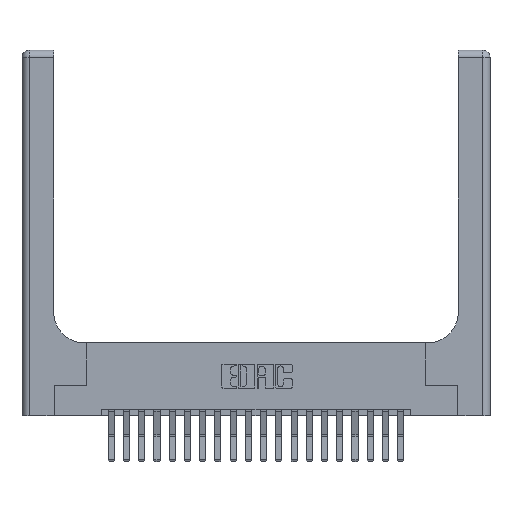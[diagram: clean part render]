
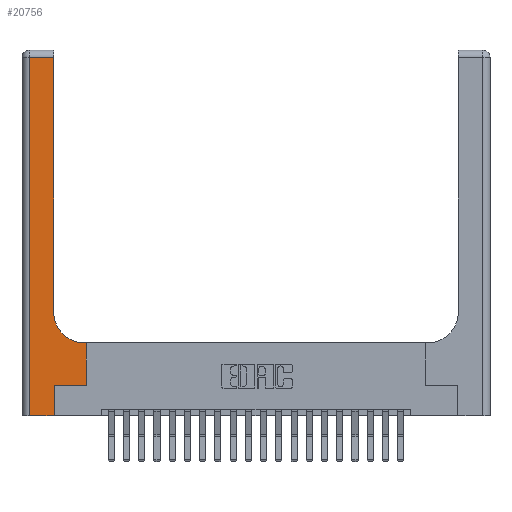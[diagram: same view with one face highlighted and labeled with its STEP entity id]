
A CAD part, top view. The second image highlights one B-rep face of the part: STEP entity #20756.
In plain terms, the highlighted planar face has unit normal (0, 0, 1).
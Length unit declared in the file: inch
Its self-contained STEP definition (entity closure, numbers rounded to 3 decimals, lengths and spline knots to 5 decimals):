
#89 = LINE ( 'NONE', #15101, #6809 ) ;
#337 = VECTOR ( 'NONE', #10274, 39.37008 ) ;
#774 = CARTESIAN_POINT ( 'NONE',  ( 0., 3., 0.37 ) ) ;
#1192 = EDGE_CURVE ( 'NONE', #19767, #1835, #10230, .T. ) ;
#1304 = VERTEX_POINT ( 'NONE', #4001 ) ;
#1382 = LINE ( 'NONE', #2144, #337 ) ;
#1524 = VERTEX_POINT ( 'NONE', #2040 ) ;
#1663 = VECTOR ( 'NONE', #15483, 39.37008 ) ;
#1835 = VERTEX_POINT ( 'NONE', #1923 ) ;
#1923 = CARTESIAN_POINT ( 'NONE',  ( 0.26, 0.85, 0.37 ) ) ;
#1961 = VECTOR ( 'NONE', #5392, 39.37008 ) ;
#2040 = CARTESIAN_POINT ( 'NONE',  ( 0.265, 0.25, 0.37 ) ) ;
#2084 = CARTESIAN_POINT ( 'NONE',  ( 0.265, 0., 0.37 ) ) ;
#2144 = CARTESIAN_POINT ( 'NONE',  ( 0., 0., 0.37 ) ) ;
#2389 = LINE ( 'NONE', #8883, #14966 ) ;
#3024 = ORIENTED_EDGE ( 'NONE', *, *, #19843, .T. ) ;
#3281 = EDGE_CURVE ( 'NONE', #1304, #16478, #4463, .T. ) ;
#3885 = ORIENTED_EDGE ( 'NONE', *, *, #8277, .T. ) ;
#4001 = CARTESIAN_POINT ( 'NONE',  ( 0.528, 0.25, 0.37 ) ) ;
#4047 = VECTOR ( 'NONE', #20188, 39.37008 ) ;
#4308 = EDGE_CURVE ( 'NONE', #13788, #12608, #2389, .T. ) ;
#4463 = LINE ( 'NONE', #16210, #19872 ) ;
#4501 = DIRECTION ( 'NONE',  ( 0., 1., 0. ) ) ;
#4838 = ORIENTED_EDGE ( 'NONE', *, *, #19431, .T. ) ;
#4858 = CARTESIAN_POINT ( 'NONE',  ( 0.51, 0.6, 0.37 ) ) ;
#5392 = DIRECTION ( 'NONE',  ( 0., 1., 0. ) ) ;
#6809 = VECTOR ( 'NONE', #13540, 39.37008 ) ;
#6857 = LINE ( 'NONE', #2084, #1961 ) ;
#6874 = LINE ( 'NONE', #20128, #4047 ) ;
#7096 = DIRECTION ( 'NONE',  ( 0., -1., 0. ) ) ;
#7355 = CARTESIAN_POINT ( 'NONE',  ( 0.26, 0.6, 0.37 ) ) ;
#8277 = EDGE_CURVE ( 'NONE', #1524, #1304, #6874, .T. ) ;
#8837 = EDGE_CURVE ( 'NONE', #13889, #1524, #6857, .T. ) ;
#8883 = CARTESIAN_POINT ( 'NONE',  ( 0.06, 3., 0.37 ) ) ;
#9096 = ORIENTED_EDGE ( 'NONE', *, *, #1192, .T. ) ;
#9409 = DIRECTION ( 'NONE',  ( 0., 0., -1. ) ) ;
#10230 = CIRCLE ( 'NONE', #12477, 0.25 ) ;
#10274 = DIRECTION ( 'NONE',  ( 1., 0., 0. ) ) ;
#10662 = DIRECTION ( 'NONE',  ( -1., 0., 0. ) ) ;
#10833 = DIRECTION ( 'NONE',  ( 1., 0., 0. ) ) ;
#10998 = CARTESIAN_POINT ( 'NONE',  ( 0.265, 0., 0.37 ) ) ;
#11542 = ORIENTED_EDGE ( 'NONE', *, *, #3281, .T. ) ;
#11955 = CARTESIAN_POINT ( 'NONE',  ( 0.26, 2.94, 0.37 ) ) ;
#12282 = DIRECTION ( 'NONE',  ( -1., 0., 0. ) ) ;
#12438 = CARTESIAN_POINT ( 'NONE',  ( 0.06, 0., 0.37 ) ) ;
#12477 = AXIS2_PLACEMENT_3D ( 'NONE', #15997, #9409, #10833 ) ;
#12608 = VERTEX_POINT ( 'NONE', #12438 ) ;
#12670 = VECTOR ( 'NONE', #10662, 39.37008 ) ;
#13058 = CARTESIAN_POINT ( 'NONE',  ( 0.528, 0.6, 0.37 ) ) ;
#13449 = LINE ( 'NONE', #7355, #12670 ) ;
#13540 = DIRECTION ( 'NONE',  ( -1., 0., 0. ) ) ;
#13788 = VERTEX_POINT ( 'NONE', #20417 ) ;
#13889 = VERTEX_POINT ( 'NONE', #10998 ) ;
#14966 = VECTOR ( 'NONE', #7096, 39.37008 ) ;
#15077 = ORIENTED_EDGE ( 'NONE', *, *, #17328, .T. ) ;
#15101 = CARTESIAN_POINT ( 'NONE',  ( 0., 2.94, 0.37 ) ) ;
#15345 = CARTESIAN_POINT ( 'NONE',  ( 0.26, 3., 0.37 ) ) ;
#15483 = DIRECTION ( 'NONE',  ( 0., 1., 0. ) ) ;
#15508 = PLANE ( 'NONE',  #19569 ) ;
#15997 = CARTESIAN_POINT ( 'NONE',  ( 0.51, 0.85, 0.37 ) ) ;
#16210 = CARTESIAN_POINT ( 'NONE',  ( 0.528, 0.25, 0.37 ) ) ;
#16283 = FACE_OUTER_BOUND ( 'NONE', #16352, .T. ) ;
#16352 = EDGE_LOOP ( 'NONE', ( #4838, #3024, #18745, #17567, #18770, #3885, #11542, #15077, #9096 ) ) ;
#16478 = VERTEX_POINT ( 'NONE', #13058 ) ;
#16623 = EDGE_CURVE ( 'NONE', #12608, #13889, #1382, .T. ) ;
#17117 = VERTEX_POINT ( 'NONE', #11955 ) ;
#17149 = DIRECTION ( 'NONE',  ( 0., 0., -1. ) ) ;
#17328 = EDGE_CURVE ( 'NONE', #16478, #19767, #13449, .T. ) ;
#17567 = ORIENTED_EDGE ( 'NONE', *, *, #16623, .T. ) ;
#18745 = ORIENTED_EDGE ( 'NONE', *, *, #4308, .T. ) ;
#18770 = ORIENTED_EDGE ( 'NONE', *, *, #8837, .T. ) ;
#19116 = LINE ( 'NONE', #15345, #1663 ) ;
#19431 = EDGE_CURVE ( 'NONE', #1835, #17117, #19116, .T. ) ;
#19569 = AXIS2_PLACEMENT_3D ( 'NONE', #774, #17149, #12282 ) ;
#19767 = VERTEX_POINT ( 'NONE', #4858 ) ;
#19843 = EDGE_CURVE ( 'NONE', #17117, #13788, #89, .T. ) ;
#19872 = VECTOR ( 'NONE', #4501, 39.37008 ) ;
#20128 = CARTESIAN_POINT ( 'NONE',  ( 0.265, 0.25, 0.37 ) ) ;
#20188 = DIRECTION ( 'NONE',  ( 1., 0., 0. ) ) ;
#20417 = CARTESIAN_POINT ( 'NONE',  ( 0.06, 2.94, 0.37 ) ) ;
#20756 = ADVANCED_FACE ( 'NONE', ( #16283 ), #15508, .F. ) ;
